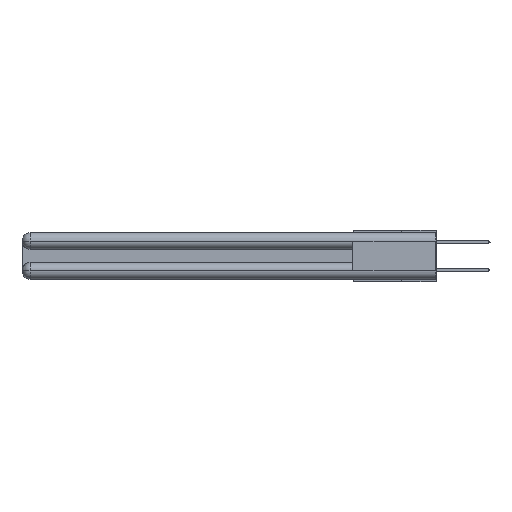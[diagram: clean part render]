
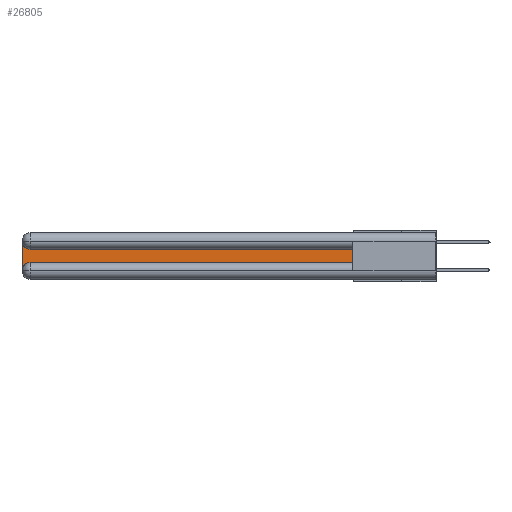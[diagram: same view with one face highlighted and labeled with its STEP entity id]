
A CAD part, left-side view. The second image highlights one B-rep face of the part: STEP entity #26805.
In plain terms, the highlighted planar face has unit normal (-1, 0, 0).
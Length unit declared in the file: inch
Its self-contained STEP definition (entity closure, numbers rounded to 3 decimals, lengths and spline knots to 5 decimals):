
#315 = CARTESIAN_POINT ( 'NONE',  ( 0.075, 0.6, -0.1225 ) ) ;
#416 = ORIENTED_EDGE ( 'NONE', *, *, #23521, .T. ) ;
#1401 = VECTOR ( 'NONE', #16646, 39.37008 ) ;
#1444 = CARTESIAN_POINT ( 'NONE',  ( 0.075, 2.94, -0.1225 ) ) ;
#1866 = CARTESIAN_POINT ( 'NONE',  ( 0.075, 2.94, -0.0625 ) ) ;
#2393 = PLANE ( 'NONE',  #3433 ) ;
#3433 = AXIS2_PLACEMENT_3D ( 'NONE', #4717, #19066, #21622 ) ;
#3444 = CARTESIAN_POINT ( 'NONE',  ( 0.075, 3., -0.2775 ) ) ;
#4034 = CIRCLE ( 'NONE', #9104, 0.06 ) ;
#4045 = LINE ( 'NONE', #11892, #1401 ) ;
#4133 = EDGE_CURVE ( 'NONE', #29977, #10694, #26441, .T. ) ;
#4267 = EDGE_LOOP ( 'NONE', ( #7143, #4835, #6479, #5357, #9611, #416 ) ) ;
#4534 = EDGE_CURVE ( 'NONE', #10694, #30806, #27169, .T. ) ;
#4717 = CARTESIAN_POINT ( 'NONE',  ( 0.075, 3., -0.1225 ) ) ;
#4835 = ORIENTED_EDGE ( 'NONE', *, *, #27759, .T. ) ;
#5357 = ORIENTED_EDGE ( 'NONE', *, *, #4534, .T. ) ;
#6479 = ORIENTED_EDGE ( 'NONE', *, *, #4133, .T. ) ;
#6621 = VERTEX_POINT ( 'NONE', #1444 ) ;
#6801 = EDGE_CURVE ( 'NONE', #30806, #28955, #4045, .T. ) ;
#7143 = ORIENTED_EDGE ( 'NONE', *, *, #10991, .T. ) ;
#9104 = AXIS2_PLACEMENT_3D ( 'NONE', #1866, #18765, #26100 ) ;
#9611 = ORIENTED_EDGE ( 'NONE', *, *, #6801, .T. ) ;
#10289 = CARTESIAN_POINT ( 'NONE',  ( 0.075, 3., -0.0625 ) ) ;
#10694 = VERTEX_POINT ( 'NONE', #3444 ) ;
#10991 = EDGE_CURVE ( 'NONE', #13755, #6621, #14000, .T. ) ;
#11017 = CARTESIAN_POINT ( 'NONE',  ( 0.075, 0.6, -0.2175 ) ) ;
#11892 = CARTESIAN_POINT ( 'NONE',  ( 0.075, 0.6, -0.2175 ) ) ;
#13755 = VERTEX_POINT ( 'NONE', #27382 ) ;
#14000 = LINE ( 'NONE', #315, #28400 ) ;
#15155 = DIRECTION ( 'NONE',  ( 0., 0., -1. ) ) ;
#16100 = FACE_OUTER_BOUND ( 'NONE', #4267, .T. ) ;
#16646 = DIRECTION ( 'NONE',  ( 0., -1., 0. ) ) ;
#16824 = CARTESIAN_POINT ( 'NONE',  ( 0.075, 3., -0.2175 ) ) ;
#18765 = DIRECTION ( 'NONE',  ( 1., 0., 0. ) ) ;
#19066 = DIRECTION ( 'NONE',  ( 1., 0., 0. ) ) ;
#19864 = DIRECTION ( 'NONE',  ( 0., 1., 0. ) ) ;
#19910 = DIRECTION ( 'NONE',  ( 1., 0., 0. ) ) ;
#20067 = LINE ( 'NONE', #31352, #21969 ) ;
#21405 = AXIS2_PLACEMENT_3D ( 'NONE', #24915, #19910, #15155 ) ;
#21622 = DIRECTION ( 'NONE',  ( 0., 0., -1. ) ) ;
#21872 = VECTOR ( 'NONE', #31315, 39.37008 ) ;
#21969 = VECTOR ( 'NONE', #26692, 39.37008 ) ;
#23521 = EDGE_CURVE ( 'NONE', #28955, #13755, #20067, .T. ) ;
#24915 = CARTESIAN_POINT ( 'NONE',  ( 0.075, 2.94, -0.2775 ) ) ;
#26100 = DIRECTION ( 'NONE',  ( 0., 0., -1. ) ) ;
#26441 = LINE ( 'NONE', #16824, #21872 ) ;
#26692 = DIRECTION ( 'NONE',  ( 0., 0., 1. ) ) ;
#26805 = ADVANCED_FACE ( 'NONE', ( #16100 ), #2393, .F. ) ;
#27169 = CIRCLE ( 'NONE', #21405, 0.06 ) ;
#27382 = CARTESIAN_POINT ( 'NONE',  ( 0.075, 0.6, -0.1225 ) ) ;
#27759 = EDGE_CURVE ( 'NONE', #6621, #29977, #4034, .T. ) ;
#28400 = VECTOR ( 'NONE', #19864, 39.37008 ) ;
#28955 = VERTEX_POINT ( 'NONE', #11017 ) ;
#29932 = CARTESIAN_POINT ( 'NONE',  ( 0.075, 2.94, -0.2175 ) ) ;
#29977 = VERTEX_POINT ( 'NONE', #10289 ) ;
#30806 = VERTEX_POINT ( 'NONE', #29932 ) ;
#31315 = DIRECTION ( 'NONE',  ( 0., 0., -1. ) ) ;
#31352 = CARTESIAN_POINT ( 'NONE',  ( 0.075, 0.6, -0.2175 ) ) ;
